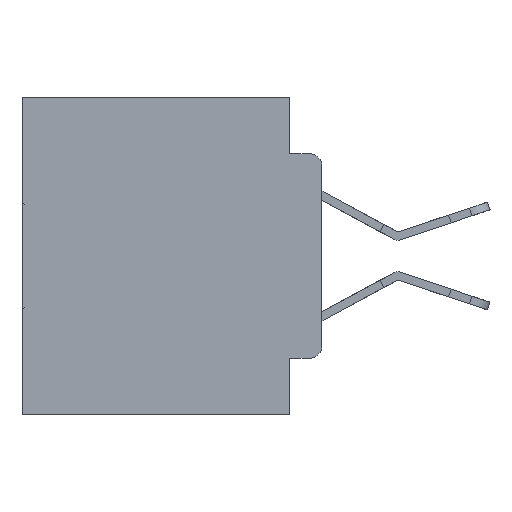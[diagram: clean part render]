
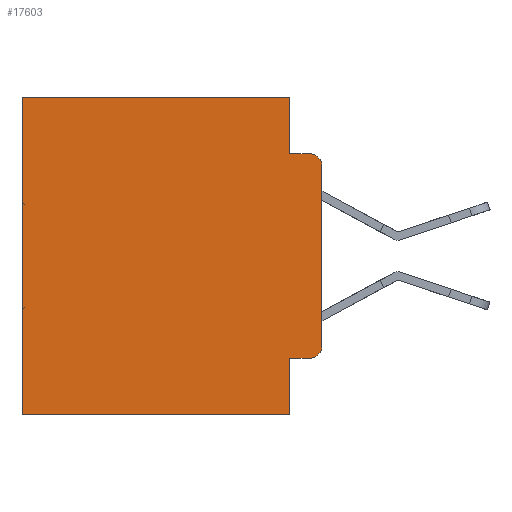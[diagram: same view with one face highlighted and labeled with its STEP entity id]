
A CAD part, left-side view. The second image highlights one B-rep face of the part: STEP entity #17603.
In plain terms, the highlighted planar face has unit normal (-1, 0, 0).
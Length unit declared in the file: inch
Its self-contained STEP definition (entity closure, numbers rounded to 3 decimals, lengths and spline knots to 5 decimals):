
#345 = PLANE ( 'NONE',  #31827 ) ;
#632 = CARTESIAN_POINT ( 'NONE',  ( 0.298, 0.051, 0. ) ) ;
#781 = ORIENTED_EDGE ( 'NONE', *, *, #4753, .T. ) ;
#953 = DIRECTION ( 'NONE',  ( 0., 0., -1. ) ) ;
#2043 = LINE ( 'NONE', #12935, #18839 ) ;
#2617 = VECTOR ( 'NONE', #953, 39.37008 ) ;
#2830 = VERTEX_POINT ( 'NONE', #5471 ) ;
#3023 = EDGE_CURVE ( 'NONE', #15886, #16303, #24858, .T. ) ;
#3480 = EDGE_CURVE ( 'NONE', #4293, #19490, #14614, .T. ) ;
#4293 = VERTEX_POINT ( 'NONE', #32074 ) ;
#4752 = CARTESIAN_POINT ( 'NONE',  ( 0.298, 0., -0.3915 ) ) ;
#4753 = EDGE_CURVE ( 'NONE', #9678, #4293, #25238, .T. ) ;
#4890 = VECTOR ( 'NONE', #13969, 39.37008 ) ;
#5471 = CARTESIAN_POINT ( 'NONE',  ( 0.298, 0.051, -0.4115 ) ) ;
#6017 = CARTESIAN_POINT ( 'NONE',  ( 0.298, 0.473, -0.5 ) ) ;
#6411 = VECTOR ( 'NONE', #29396, 39.37008 ) ;
#6485 = ORIENTED_EDGE ( 'NONE', *, *, #27563, .T. ) ;
#7214 = VERTEX_POINT ( 'NONE', #11373 ) ;
#7730 = DIRECTION ( 'NONE',  ( -1., 0., 0. ) ) ;
#7948 = VERTEX_POINT ( 'NONE', #16828 ) ;
#8896 = CARTESIAN_POINT ( 'NONE',  ( 0.298, 0., -0.5 ) ) ;
#9167 = CARTESIAN_POINT ( 'NONE',  ( 0.298, 0.02, -0.0885 ) ) ;
#9657 = EDGE_CURVE ( 'NONE', #9678, #7948, #16230, .T. ) ;
#9678 = VERTEX_POINT ( 'NONE', #16158 ) ;
#10529 = CARTESIAN_POINT ( 'NONE',  ( 0.298, 0.02, -0.1085 ) ) ;
#10674 = CIRCLE ( 'NONE', #30899, 0.02 ) ;
#10750 = DIRECTION ( 'NONE',  ( 0., 1., 0. ) ) ;
#11373 = CARTESIAN_POINT ( 'NONE',  ( 0.298, 0.02, -0.4115 ) ) ;
#12935 = CARTESIAN_POINT ( 'NONE',  ( 0.298, 0.051, -0.4115 ) ) ;
#13888 = ORIENTED_EDGE ( 'NONE', *, *, #21967, .F. ) ;
#13969 = DIRECTION ( 'NONE',  ( 0., 0., -1. ) ) ;
#14023 = CARTESIAN_POINT ( 'NONE',  ( 0.298, 0.051, -0.5 ) ) ;
#14117 = ORIENTED_EDGE ( 'NONE', *, *, #14374, .F. ) ;
#14374 = EDGE_CURVE ( 'NONE', #2830, #24398, #22055, .T. ) ;
#14614 = LINE ( 'NONE', #17387, #32928 ) ;
#15247 = VECTOR ( 'NONE', #18484, 39.37008 ) ;
#15436 = DIRECTION ( 'NONE',  ( 0., 0., -1. ) ) ;
#15886 = VERTEX_POINT ( 'NONE', #31336 ) ;
#15910 = CARTESIAN_POINT ( 'NONE',  ( 0.298, 0.051, 0. ) ) ;
#16158 = CARTESIAN_POINT ( 'NONE',  ( 0.298, 0.051, 0. ) ) ;
#16230 = LINE ( 'NONE', #632, #2617 ) ;
#16303 = VERTEX_POINT ( 'NONE', #4752 ) ;
#16664 = LINE ( 'NONE', #17515, #30972 ) ;
#16826 = CIRCLE ( 'NONE', #22323, 0.02 ) ;
#16828 = CARTESIAN_POINT ( 'NONE',  ( 0.298, 0.051, -0.0885 ) ) ;
#17168 = EDGE_LOOP ( 'NONE', ( #24756, #28545, #23603, #21999, #781, #18014, #13888, #14117, #6485, #31962 ) ) ;
#17387 = CARTESIAN_POINT ( 'NONE',  ( 0.298, 0.473, 0. ) ) ;
#17448 = CARTESIAN_POINT ( 'NONE',  ( 0.298, 0.02, -0.3915 ) ) ;
#17515 = CARTESIAN_POINT ( 'NONE',  ( 0.298, 0.051, -0.0885 ) ) ;
#17603 = ADVANCED_FACE ( 'NONE', ( #19109 ), #345, .F. ) ;
#18014 = ORIENTED_EDGE ( 'NONE', *, *, #3480, .T. ) ;
#18118 = DIRECTION ( 'NONE',  ( 1., 0., 0. ) ) ;
#18280 = DIRECTION ( 'NONE',  ( 0., -1., 0. ) ) ;
#18484 = DIRECTION ( 'NONE',  ( 0., 0., -1. ) ) ;
#18839 = VECTOR ( 'NONE', #18280, 39.37008 ) ;
#19109 = FACE_OUTER_BOUND ( 'NONE', #17168, .T. ) ;
#19135 = VERTEX_POINT ( 'NONE', #9167 ) ;
#19490 = VERTEX_POINT ( 'NONE', #6017 ) ;
#19769 = DIRECTION ( 'NONE',  ( -1., 0., 0. ) ) ;
#20040 = DIRECTION ( 'NONE',  ( 0., 0., -1. ) ) ;
#21967 = EDGE_CURVE ( 'NONE', #24398, #19490, #23180, .T. ) ;
#21999 = ORIENTED_EDGE ( 'NONE', *, *, #9657, .F. ) ;
#22055 = LINE ( 'NONE', #15910, #15247 ) ;
#22323 = AXIS2_PLACEMENT_3D ( 'NONE', #10529, #7730, #25566 ) ;
#23180 = LINE ( 'NONE', #8896, #6411 ) ;
#23327 = EDGE_CURVE ( 'NONE', #7214, #16303, #10674, .T. ) ;
#23461 = CARTESIAN_POINT ( 'NONE',  ( 0.298, 0., 0. ) ) ;
#23603 = ORIENTED_EDGE ( 'NONE', *, *, #24009, .F. ) ;
#24009 = EDGE_CURVE ( 'NONE', #7948, #19135, #16664, .T. ) ;
#24398 = VERTEX_POINT ( 'NONE', #14023 ) ;
#24756 = ORIENTED_EDGE ( 'NONE', *, *, #3023, .F. ) ;
#24849 = VECTOR ( 'NONE', #10750, 39.37008 ) ;
#24858 = LINE ( 'NONE', #26866, #4890 ) ;
#25238 = LINE ( 'NONE', #23461, #24849 ) ;
#25566 = DIRECTION ( 'NONE',  ( 0., 0., -1. ) ) ;
#25975 = CARTESIAN_POINT ( 'NONE',  ( 0.298, 0., 0. ) ) ;
#26866 = CARTESIAN_POINT ( 'NONE',  ( 0.298, 0., 0. ) ) ;
#27563 = EDGE_CURVE ( 'NONE', #2830, #7214, #2043, .T. ) ;
#27681 = DIRECTION ( 'NONE',  ( 0., -1., 0. ) ) ;
#28189 = EDGE_CURVE ( 'NONE', #15886, #19135, #16826, .T. ) ;
#28545 = ORIENTED_EDGE ( 'NONE', *, *, #28189, .T. ) ;
#29396 = DIRECTION ( 'NONE',  ( 0., 1., 0. ) ) ;
#29864 = DIRECTION ( 'NONE',  ( 0., 0., -1. ) ) ;
#30899 = AXIS2_PLACEMENT_3D ( 'NONE', #17448, #19769, #29864 ) ;
#30972 = VECTOR ( 'NONE', #27681, 39.37008 ) ;
#31336 = CARTESIAN_POINT ( 'NONE',  ( 0.298, 0., -0.1085 ) ) ;
#31827 = AXIS2_PLACEMENT_3D ( 'NONE', #25975, #18118, #15436 ) ;
#31962 = ORIENTED_EDGE ( 'NONE', *, *, #23327, .T. ) ;
#32074 = CARTESIAN_POINT ( 'NONE',  ( 0.298, 0.473, 0. ) ) ;
#32928 = VECTOR ( 'NONE', #20040, 39.37008 ) ;
